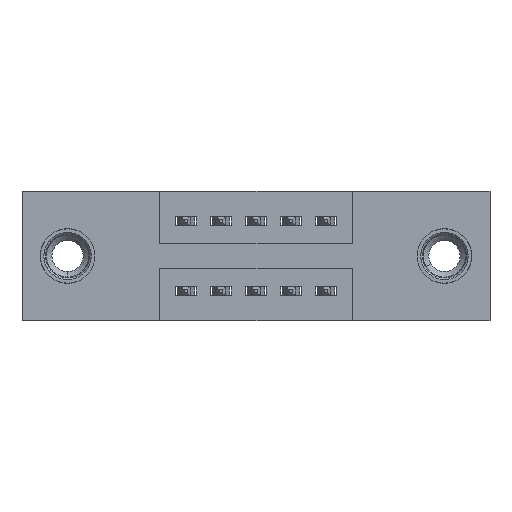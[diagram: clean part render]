
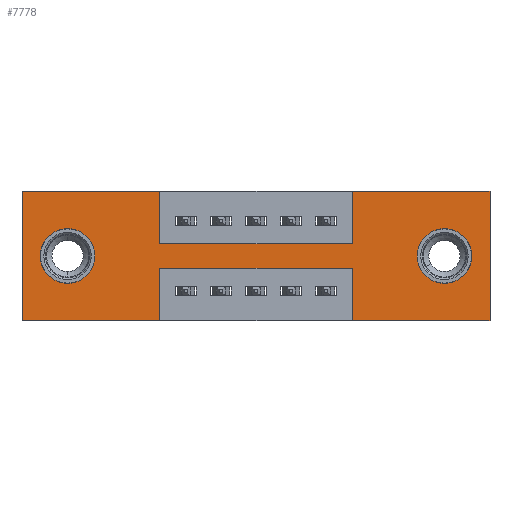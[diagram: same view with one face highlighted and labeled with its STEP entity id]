
A CAD part, front view. The second image highlights one B-rep face of the part: STEP entity #7778.
In plain terms, the highlighted planar face has unit normal (0, -1, 0).
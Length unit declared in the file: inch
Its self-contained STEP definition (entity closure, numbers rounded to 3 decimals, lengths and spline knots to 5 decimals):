
#21 = CARTESIAN_POINT ( 'NONE',  ( 0., 0., -0.37 ) ) ;
#95 = VECTOR ( 'NONE', #6967, 39.37008 ) ;
#101 = VERTEX_POINT ( 'NONE', #9916 ) ;
#107 = EDGE_CURVE ( 'NONE', #6640, #101, #9226, .T. ) ;
#187 = CARTESIAN_POINT ( 'NONE',  ( 1.335, 0., -0.37 ) ) ;
#205 = CARTESIAN_POINT ( 'NONE',  ( 0.13, 0., -0.107 ) ) ;
#236 = LINE ( 'NONE', #2966, #9641 ) ;
#281 = CARTESIAN_POINT ( 'NONE',  ( 0., 0., -0.37 ) ) ;
#338 = LINE ( 'NONE', #281, #6200 ) ;
#361 = ORIENTED_EDGE ( 'NONE', *, *, #9599, .T. ) ;
#409 = ORIENTED_EDGE ( 'NONE', *, *, #6691, .F. ) ;
#439 = DIRECTION ( 'NONE',  ( 0., 0., 1. ) ) ;
#488 = VECTOR ( 'NONE', #4437, 39.37008 ) ;
#542 = EDGE_CURVE ( 'NONE', #8556, #3961, #9680, .T. ) ;
#617 = VERTEX_POINT ( 'NONE', #7408 ) ;
#696 = ORIENTED_EDGE ( 'NONE', *, *, #9721, .F. ) ;
#764 = LINE ( 'NONE', #4046, #8838 ) ;
#820 = CARTESIAN_POINT ( 'NONE',  ( 0.3925, 0., -0.15 ) ) ;
#855 = CARTESIAN_POINT ( 'NONE',  ( 0., 0., -0.37 ) ) ;
#893 = VERTEX_POINT ( 'NONE', #2001 ) ;
#964 = FACE_BOUND ( 'NONE', #7758, .T. ) ;
#1084 = VERTEX_POINT ( 'NONE', #8922 ) ;
#1085 = VERTEX_POINT ( 'NONE', #8732 ) ;
#1200 = FACE_BOUND ( 'NONE', #2230, .T. ) ;
#1255 = EDGE_CURVE ( 'NONE', #1084, #893, #3895, .T. ) ;
#1257 = AXIS2_PLACEMENT_3D ( 'NONE', #8880, #4258, #9625 ) ;
#1318 = CARTESIAN_POINT ( 'NONE',  ( 0.3925, 0., -0.22 ) ) ;
#1319 = VECTOR ( 'NONE', #9268, 39.37008 ) ;
#1525 = VECTOR ( 'NONE', #9046, 39.37008 ) ;
#1580 = VECTOR ( 'NONE', #8353, 39.37008 ) ;
#1595 = DIRECTION ( 'NONE',  ( 0., 1., 0. ) ) ;
#1668 = VERTEX_POINT ( 'NONE', #4855 ) ;
#1720 = CARTESIAN_POINT ( 'NONE',  ( 0., 0., 0. ) ) ;
#2001 = CARTESIAN_POINT ( 'NONE',  ( 1.335, 0., 0. ) ) ;
#2035 = VECTOR ( 'NONE', #5634, 39.37008 ) ;
#2230 = EDGE_LOOP ( 'NONE', ( #3469, #2746 ) ) ;
#2261 = CARTESIAN_POINT ( 'NONE',  ( 0.3925, 0., -0.15 ) ) ;
#2292 = EDGE_CURVE ( 'NONE', #617, #8556, #764, .T. ) ;
#2348 = ORIENTED_EDGE ( 'NONE', *, *, #7513, .F. ) ;
#2472 = CARTESIAN_POINT ( 'NONE',  ( 0.13, 0., -0.185 ) ) ;
#2576 = EDGE_CURVE ( 'NONE', #3961, #8384, #4366, .T. ) ;
#2691 = DIRECTION ( 'NONE',  ( -1., 0., 0. ) ) ;
#2746 = ORIENTED_EDGE ( 'NONE', *, *, #6263, .T. ) ;
#2846 = VERTEX_POINT ( 'NONE', #9869 ) ;
#2849 = LINE ( 'NONE', #4435, #488 ) ;
#2932 = CARTESIAN_POINT ( 'NONE',  ( 1.205, 0., -0.263 ) ) ;
#2966 = CARTESIAN_POINT ( 'NONE',  ( 0.9425, 0., -0.37 ) ) ;
#3022 = CARTESIAN_POINT ( 'NONE',  ( 0.3925, 0., -0.37 ) ) ;
#3104 = VERTEX_POINT ( 'NONE', #205 ) ;
#3190 = EDGE_CURVE ( 'NONE', #8103, #6082, #2849, .T. ) ;
#3292 = DIRECTION ( 'NONE',  ( 0., 0., 1. ) ) ;
#3293 = VERTEX_POINT ( 'NONE', #6216 ) ;
#3315 = EDGE_CURVE ( 'NONE', #893, #5228, #5850, .T. ) ;
#3332 = DIRECTION ( 'NONE',  ( 0., -1., 0. ) ) ;
#3369 = AXIS2_PLACEMENT_3D ( 'NONE', #21, #3332, #8757 ) ;
#3469 = ORIENTED_EDGE ( 'NONE', *, *, #6707, .T. ) ;
#3574 = CARTESIAN_POINT ( 'NONE',  ( 0.3925, 0., 0. ) ) ;
#3708 = DIRECTION ( 'NONE',  ( 0., 0., -1. ) ) ;
#3754 = DIRECTION ( 'NONE',  ( 0., 0., 1. ) ) ;
#3783 = AXIS2_PLACEMENT_3D ( 'NONE', #6377, #1595, #9203 ) ;
#3861 = ORIENTED_EDGE ( 'NONE', *, *, #542, .F. ) ;
#3895 = LINE ( 'NONE', #8265, #7311 ) ;
#3922 = EDGE_CURVE ( 'NONE', #6082, #617, #338, .T. ) ;
#3961 = VERTEX_POINT ( 'NONE', #3574 ) ;
#3968 = LINE ( 'NONE', #9770, #6089 ) ;
#4046 = CARTESIAN_POINT ( 'NONE',  ( 0., 0., 0. ) ) ;
#4258 = DIRECTION ( 'NONE',  ( 0., 1., 0. ) ) ;
#4366 = LINE ( 'NONE', #6991, #95 ) ;
#4435 = CARTESIAN_POINT ( 'NONE',  ( 0.3925, 0., -0.37 ) ) ;
#4437 = DIRECTION ( 'NONE',  ( 0., 0., -1. ) ) ;
#4580 = DIRECTION ( 'NONE',  ( 0., 0., 1. ) ) ;
#4855 = CARTESIAN_POINT ( 'NONE',  ( 0.9425, 0., -0.37 ) ) ;
#4909 = DIRECTION ( 'NONE',  ( 1., 0., 0. ) ) ;
#4942 = EDGE_CURVE ( 'NONE', #8384, #2846, #7600, .T. ) ;
#5122 = EDGE_LOOP ( 'NONE', ( #8375, #696, #409, #6784, #7243, #5189, #2348, #6914, #8661, #3861, #6454, #5464 ) ) ;
#5189 = ORIENTED_EDGE ( 'NONE', *, *, #1255, .F. ) ;
#5228 = VERTEX_POINT ( 'NONE', #187 ) ;
#5464 = ORIENTED_EDGE ( 'NONE', *, *, #3922, .F. ) ;
#5634 = DIRECTION ( 'NONE',  ( -1., 0., 0. ) ) ;
#5643 = AXIS2_PLACEMENT_3D ( 'NONE', #8647, #8261, #3708 ) ;
#5850 = LINE ( 'NONE', #7157, #1580 ) ;
#5863 = CARTESIAN_POINT ( 'NONE',  ( 0., 0., 0. ) ) ;
#6040 = CARTESIAN_POINT ( 'NONE',  ( 0.3925, 0., -0.22 ) ) ;
#6082 = VERTEX_POINT ( 'NONE', #3022 ) ;
#6089 = VECTOR ( 'NONE', #439, 39.37008 ) ;
#6200 = VECTOR ( 'NONE', #2691, 39.37008 ) ;
#6216 = CARTESIAN_POINT ( 'NONE',  ( 0.13, 0., -0.263 ) ) ;
#6248 = EDGE_CURVE ( 'NONE', #5228, #1668, #6282, .T. ) ;
#6263 = EDGE_CURVE ( 'NONE', #3293, #3104, #8289, .T. ) ;
#6282 = LINE ( 'NONE', #855, #2035 ) ;
#6377 = CARTESIAN_POINT ( 'NONE',  ( 1.205, 0., -0.185 ) ) ;
#6454 = ORIENTED_EDGE ( 'NONE', *, *, #2292, .F. ) ;
#6640 = VERTEX_POINT ( 'NONE', #2932 ) ;
#6691 = EDGE_CURVE ( 'NONE', #1668, #1085, #236, .T. ) ;
#6707 = EDGE_CURVE ( 'NONE', #3104, #3293, #9410, .T. ) ;
#6784 = ORIENTED_EDGE ( 'NONE', *, *, #6248, .F. ) ;
#6914 = ORIENTED_EDGE ( 'NONE', *, *, #4942, .F. ) ;
#6967 = DIRECTION ( 'NONE',  ( 0., 0., -1. ) ) ;
#6991 = CARTESIAN_POINT ( 'NONE',  ( 0.3925, 0., 0. ) ) ;
#7157 = CARTESIAN_POINT ( 'NONE',  ( 1.335, 0., 0. ) ) ;
#7243 = ORIENTED_EDGE ( 'NONE', *, *, #3315, .F. ) ;
#7252 = FACE_OUTER_BOUND ( 'NONE', #5122, .T. ) ;
#7311 = VECTOR ( 'NONE', #7972, 39.37008 ) ;
#7408 = CARTESIAN_POINT ( 'NONE',  ( 0., 0., -0.37 ) ) ;
#7513 = EDGE_CURVE ( 'NONE', #2846, #1084, #3968, .T. ) ;
#7600 = LINE ( 'NONE', #2261, #1319 ) ;
#7758 = EDGE_LOOP ( 'NONE', ( #361, #9180 ) ) ;
#7778 = ADVANCED_FACE ( 'NONE', ( #964, #1200, #7252 ), #7988, .T. ) ;
#7802 = LINE ( 'NONE', #6040, #1525 ) ;
#7945 = DIRECTION ( 'NONE',  ( 0., 1., 0. ) ) ;
#7972 = DIRECTION ( 'NONE',  ( 1., 0., 0. ) ) ;
#7988 = PLANE ( 'NONE',  #3369 ) ;
#8103 = VERTEX_POINT ( 'NONE', #1318 ) ;
#8261 = DIRECTION ( 'NONE',  ( 0., 1., 0. ) ) ;
#8265 = CARTESIAN_POINT ( 'NONE',  ( 0., 0., 0. ) ) ;
#8289 = CIRCLE ( 'NONE', #9486, 0.078 ) ;
#8353 = DIRECTION ( 'NONE',  ( 0., 0., -1. ) ) ;
#8375 = ORIENTED_EDGE ( 'NONE', *, *, #3190, .F. ) ;
#8384 = VERTEX_POINT ( 'NONE', #820 ) ;
#8395 = VECTOR ( 'NONE', #4909, 39.37008 ) ;
#8556 = VERTEX_POINT ( 'NONE', #5863 ) ;
#8647 = CARTESIAN_POINT ( 'NONE',  ( 1.205, 0., -0.185 ) ) ;
#8661 = ORIENTED_EDGE ( 'NONE', *, *, #2576, .F. ) ;
#8732 = CARTESIAN_POINT ( 'NONE',  ( 0.9425, 0., -0.22 ) ) ;
#8757 = DIRECTION ( 'NONE',  ( 0., 0., -1. ) ) ;
#8761 = CIRCLE ( 'NONE', #3783, 0.078 ) ;
#8838 = VECTOR ( 'NONE', #3754, 39.37008 ) ;
#8880 = CARTESIAN_POINT ( 'NONE',  ( 0.13, 0., -0.185 ) ) ;
#8922 = CARTESIAN_POINT ( 'NONE',  ( 0.9425, 0., 0. ) ) ;
#9046 = DIRECTION ( 'NONE',  ( -1., 0., 0. ) ) ;
#9180 = ORIENTED_EDGE ( 'NONE', *, *, #107, .T. ) ;
#9203 = DIRECTION ( 'NONE',  ( 0., 0., -1. ) ) ;
#9226 = CIRCLE ( 'NONE', #5643, 0.078 ) ;
#9268 = DIRECTION ( 'NONE',  ( 1., 0., 0. ) ) ;
#9410 = CIRCLE ( 'NONE', #1257, 0.078 ) ;
#9486 = AXIS2_PLACEMENT_3D ( 'NONE', #2472, #7945, #3292 ) ;
#9599 = EDGE_CURVE ( 'NONE', #101, #6640, #8761, .T. ) ;
#9625 = DIRECTION ( 'NONE',  ( 0., 0., 1. ) ) ;
#9641 = VECTOR ( 'NONE', #4580, 39.37008 ) ;
#9680 = LINE ( 'NONE', #1720, #8395 ) ;
#9721 = EDGE_CURVE ( 'NONE', #1085, #8103, #7802, .T. ) ;
#9770 = CARTESIAN_POINT ( 'NONE',  ( 0.9425, 0., 0. ) ) ;
#9869 = CARTESIAN_POINT ( 'NONE',  ( 0.9425, 0., -0.15 ) ) ;
#9916 = CARTESIAN_POINT ( 'NONE',  ( 1.205, 0., -0.107 ) ) ;
